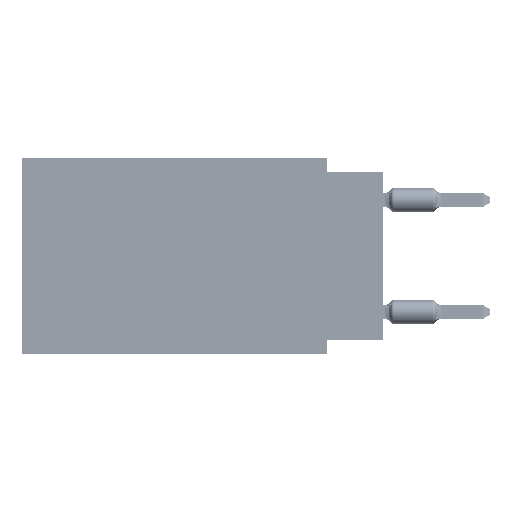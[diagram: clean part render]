
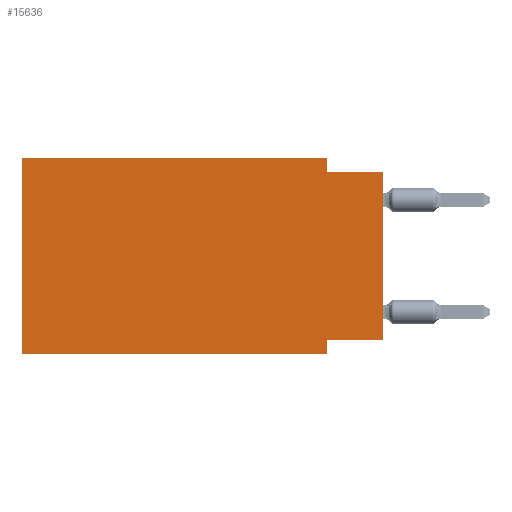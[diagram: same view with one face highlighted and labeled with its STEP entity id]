
A CAD part, left-side view. The second image highlights one B-rep face of the part: STEP entity #15636.
In plain terms, the highlighted planar face has unit normal (-1, 0, 0).
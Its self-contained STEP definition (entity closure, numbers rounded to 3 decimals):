
#1642 = VERTEX_POINT ( 'NONE', #49505 ) ;
#1841 = EDGE_CURVE ( 'NONE', #61858, #57619, #47656, .T. ) ;
#2000 = LINE ( 'NONE', #52313, #48642 ) ;
#2067 = CARTESIAN_POINT ( 'NONE',  ( 0., 16.383, -8.89 ) ) ;
#2286 = DIRECTION ( 'NONE',  ( 0., -1., 0. ) ) ;
#5650 = DIRECTION ( 'NONE',  ( 0., 1., 0. ) ) ;
#8424 = VECTOR ( 'NONE', #48016, 1000. ) ;
#8576 = VECTOR ( 'NONE', #36161, 1000. ) ;
#11265 = CARTESIAN_POINT ( 'NONE',  ( 0., 0., -0.635 ) ) ;
#12564 = CARTESIAN_POINT ( 'NONE',  ( 0., 16.383, 0. ) ) ;
#14726 = ORIENTED_EDGE ( 'NONE', *, *, #15393, .T. ) ;
#15393 = EDGE_CURVE ( 'NONE', #61057, #22335, #70126, .T. ) ;
#15636 = ADVANCED_FACE ( 'NONE', ( #66851 ), #45282, .F. ) ;
#17714 = EDGE_CURVE ( 'NONE', #57619, #30379, #31127, .T. ) ;
#19247 = VECTOR ( 'NONE', #64371, 1000. ) ;
#19509 = ORIENTED_EDGE ( 'NONE', *, *, #61694, .F. ) ;
#21854 = LINE ( 'NONE', #44482, #66176 ) ;
#22176 = ORIENTED_EDGE ( 'NONE', *, *, #58230, .F. ) ;
#22335 = VERTEX_POINT ( 'NONE', #37245 ) ;
#23404 = ORIENTED_EDGE ( 'NONE', *, *, #1841, .F. ) ;
#26104 = CARTESIAN_POINT ( 'NONE',  ( 0., 2.54, 0. ) ) ;
#29589 = CARTESIAN_POINT ( 'NONE',  ( 0., 16.383, 0. ) ) ;
#30379 = VERTEX_POINT ( 'NONE', #57686 ) ;
#31127 = LINE ( 'NONE', #26104, #8424 ) ;
#35610 = EDGE_CURVE ( 'NONE', #30379, #40461, #51536, .T. ) ;
#36161 = DIRECTION ( 'NONE',  ( 0., -1., 0. ) ) ;
#36897 = VECTOR ( 'NONE', #59844, 1000. ) ;
#37245 = CARTESIAN_POINT ( 'NONE',  ( 0., 2.54, -8.89 ) ) ;
#37435 = CARTESIAN_POINT ( 'NONE',  ( 0., 16.383, -8.89 ) ) ;
#37586 = LINE ( 'NONE', #59496, #36897 ) ;
#38228 = VECTOR ( 'NONE', #49041, 1000. ) ;
#39548 = DIRECTION ( 'NONE',  ( 1., 0., 0. ) ) ;
#40216 = VERTEX_POINT ( 'NONE', #66383 ) ;
#40461 = VERTEX_POINT ( 'NONE', #11265 ) ;
#41111 = EDGE_CURVE ( 'NONE', #1642, #40216, #21854, .T. ) ;
#41538 = DIRECTION ( 'NONE',  ( 0., 0., 1. ) ) ;
#41554 = CARTESIAN_POINT ( 'NONE',  ( 0., 16.383, 0. ) ) ;
#44482 = CARTESIAN_POINT ( 'NONE',  ( 0., 0., -8.255 ) ) ;
#45282 = PLANE ( 'NONE',  #69731 ) ;
#47351 = ORIENTED_EDGE ( 'NONE', *, *, #17714, .F. ) ;
#47656 = LINE ( 'NONE', #41554, #8576 ) ;
#48016 = DIRECTION ( 'NONE',  ( 0., 0., -1. ) ) ;
#48642 = VECTOR ( 'NONE', #41538, 1000. ) ;
#49041 = DIRECTION ( 'NONE',  ( 0., 0., 1. ) ) ;
#49054 = ORIENTED_EDGE ( 'NONE', *, *, #62625, .T. ) ;
#49505 = CARTESIAN_POINT ( 'NONE',  ( 0., 0., -8.255 ) ) ;
#51536 = LINE ( 'NONE', #62667, #67393 ) ;
#52313 = CARTESIAN_POINT ( 'NONE',  ( 0., 0., 0. ) ) ;
#52772 = CARTESIAN_POINT ( 'NONE',  ( 0., 2.54, 0. ) ) ;
#54432 = CARTESIAN_POINT ( 'NONE',  ( 0., 16.383, 0. ) ) ;
#57619 = VERTEX_POINT ( 'NONE', #52772 ) ;
#57686 = CARTESIAN_POINT ( 'NONE',  ( 0., 2.54, -0.635 ) ) ;
#58230 = EDGE_CURVE ( 'NONE', #40216, #22335, #37586, .T. ) ;
#59496 = CARTESIAN_POINT ( 'NONE',  ( 0., 2.54, -8.89 ) ) ;
#59844 = DIRECTION ( 'NONE',  ( 0., 0., -1. ) ) ;
#61057 = VERTEX_POINT ( 'NONE', #2067 ) ;
#61459 = DIRECTION ( 'NONE',  ( 0., 0., -1. ) ) ;
#61694 = EDGE_CURVE ( 'NONE', #61057, #61858, #66264, .T. ) ;
#61858 = VERTEX_POINT ( 'NONE', #29589 ) ;
#61939 = EDGE_LOOP ( 'NONE', ( #49054, #70328, #47351, #23404, #19509, #14726, #22176, #63385 ) ) ;
#62625 = EDGE_CURVE ( 'NONE', #1642, #40461, #2000, .T. ) ;
#62667 = CARTESIAN_POINT ( 'NONE',  ( 0., 0., -0.635 ) ) ;
#63385 = ORIENTED_EDGE ( 'NONE', *, *, #41111, .F. ) ;
#64371 = DIRECTION ( 'NONE',  ( 0., -1., 0. ) ) ;
#66176 = VECTOR ( 'NONE', #5650, 1000. ) ;
#66264 = LINE ( 'NONE', #54432, #38228 ) ;
#66383 = CARTESIAN_POINT ( 'NONE',  ( 0., 2.54, -8.255 ) ) ;
#66851 = FACE_OUTER_BOUND ( 'NONE', #61939, .T. ) ;
#67393 = VECTOR ( 'NONE', #2286, 1000. ) ;
#69731 = AXIS2_PLACEMENT_3D ( 'NONE', #12564, #39548, #61459 ) ;
#70126 = LINE ( 'NONE', #37435, #19247 ) ;
#70328 = ORIENTED_EDGE ( 'NONE', *, *, #35610, .F. ) ;
